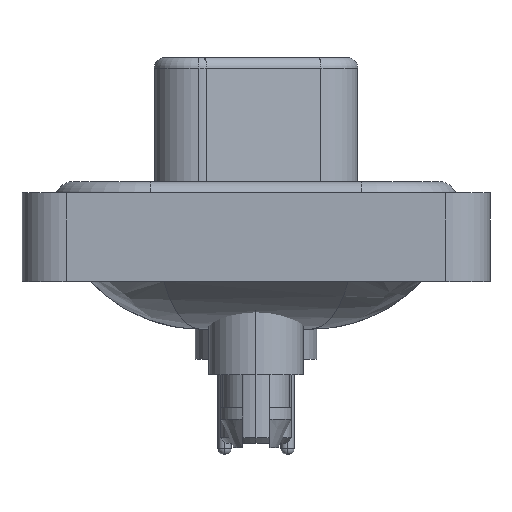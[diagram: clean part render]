
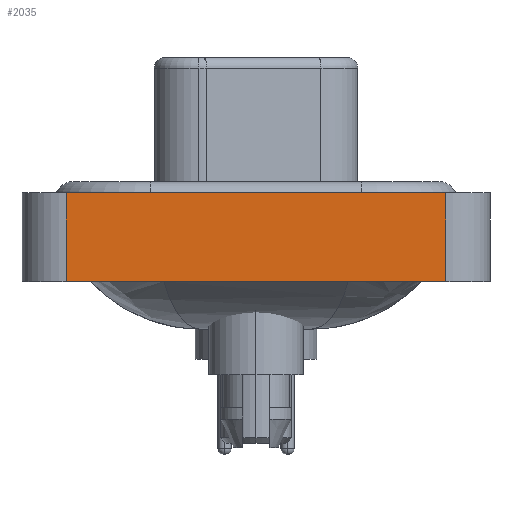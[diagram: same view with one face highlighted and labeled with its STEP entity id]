
A CAD part, left-side view. The second image highlights one B-rep face of the part: STEP entity #2035.
In plain terms, the highlighted planar face has unit normal (-1, 0, 0).
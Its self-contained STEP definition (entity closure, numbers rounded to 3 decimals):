
#1029 = VECTOR ( 'NONE', #13560, 1000. ) ;
#2035 = ADVANCED_FACE ( 'NONE', ( #8216 ), #16137, .T. ) ;
#2880 = DIRECTION ( 'NONE',  ( 0., -1., 0. ) ) ;
#4622 = EDGE_LOOP ( 'NONE', ( #15085, #12444, #17076, #19367 ) ) ;
#5649 = CARTESIAN_POINT ( 'NONE',  ( -7.35, 8.55, -3.6 ) ) ;
#5954 = AXIS2_PLACEMENT_3D ( 'NONE', #24100, #14172, #19668 ) ;
#6639 = LINE ( 'NONE', #14824, #15700 ) ;
#8216 = FACE_OUTER_BOUND ( 'NONE', #4622, .T. ) ;
#8635 = LINE ( 'NONE', #20744, #20254 ) ;
#9647 = CARTESIAN_POINT ( 'NONE',  ( -7.35, 8.55, -3.6 ) ) ;
#9667 = VERTEX_POINT ( 'NONE', #25533 ) ;
#9723 = EDGE_CURVE ( 'NONE', #9667, #23285, #6639, .T. ) ;
#12397 = EDGE_CURVE ( 'NONE', #25746, #23285, #22818, .T. ) ;
#12444 = ORIENTED_EDGE ( 'NONE', *, *, #12397, .F. ) ;
#12604 = DIRECTION ( 'NONE',  ( 0., 0., 1. ) ) ;
#12694 = VERTEX_POINT ( 'NONE', #9647 ) ;
#13560 = DIRECTION ( 'NONE',  ( 0., 0., 1. ) ) ;
#14172 = DIRECTION ( 'NONE',  ( -1., 0., 0. ) ) ;
#14582 = CARTESIAN_POINT ( 'NONE',  ( -7.35, -8.55, 0.4 ) ) ;
#14824 = CARTESIAN_POINT ( 'NONE',  ( -7.35, -8.55, -3.6 ) ) ;
#15085 = ORIENTED_EDGE ( 'NONE', *, *, #9723, .T. ) ;
#15700 = VECTOR ( 'NONE', #12604, 1000. ) ;
#16137 = PLANE ( 'NONE',  #5954 ) ;
#17076 = ORIENTED_EDGE ( 'NONE', *, *, #22906, .F. ) ;
#19111 = CARTESIAN_POINT ( 'NONE',  ( -7.35, -8.55, 0.4 ) ) ;
#19153 = CARTESIAN_POINT ( 'NONE',  ( -7.35, 8.55, 0.4 ) ) ;
#19367 = ORIENTED_EDGE ( 'NONE', *, *, #25603, .T. ) ;
#19668 = DIRECTION ( 'NONE',  ( 0., 0., 1. ) ) ;
#20254 = VECTOR ( 'NONE', #2880, 1000. ) ;
#20744 = CARTESIAN_POINT ( 'NONE',  ( -7.35, -8.55, -3.6 ) ) ;
#22818 = LINE ( 'NONE', #14582, #23930 ) ;
#22906 = EDGE_CURVE ( 'NONE', #12694, #25746, #25422, .T. ) ;
#23285 = VERTEX_POINT ( 'NONE', #19111 ) ;
#23930 = VECTOR ( 'NONE', #24385, 1000. ) ;
#24100 = CARTESIAN_POINT ( 'NONE',  ( -7.35, -8.55, -3.6 ) ) ;
#24385 = DIRECTION ( 'NONE',  ( 0., -1., 0. ) ) ;
#25422 = LINE ( 'NONE', #5649, #1029 ) ;
#25533 = CARTESIAN_POINT ( 'NONE',  ( -7.35, -8.55, -3.6 ) ) ;
#25603 = EDGE_CURVE ( 'NONE', #12694, #9667, #8635, .T. ) ;
#25746 = VERTEX_POINT ( 'NONE', #19153 ) ;
